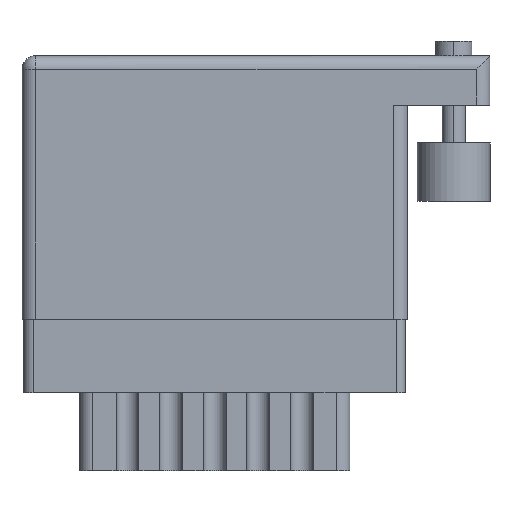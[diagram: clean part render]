
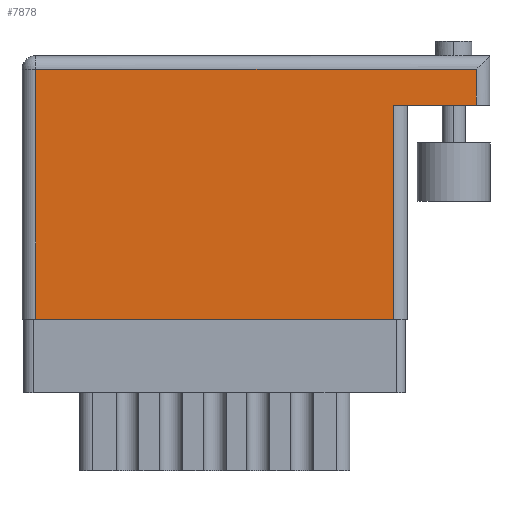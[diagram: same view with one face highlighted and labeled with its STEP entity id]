
A CAD part, front view. The second image highlights one B-rep face of the part: STEP entity #7878.
In plain terms, the highlighted face is planar.
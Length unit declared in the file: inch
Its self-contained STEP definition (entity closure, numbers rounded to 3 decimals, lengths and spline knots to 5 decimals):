
#89 = EDGE_CURVE ( 'NONE', #20875, #8784, #2926, .T. ) ;
#246 = DIRECTION ( 'NONE',  ( 0., 1., 0. ) ) ;
#367 = ORIENTED_EDGE ( 'NONE', *, *, #19739, .T. ) ;
#633 = DIRECTION ( 'NONE',  ( -1., 0., 0. ) ) ;
#801 = VERTEX_POINT ( 'NONE', #1222 ) ;
#1222 = CARTESIAN_POINT ( 'NONE',  ( 1.278, 0.736, 0. ) ) ;
#1273 = ORIENTED_EDGE ( 'NONE', *, *, #17469, .T. ) ;
#1598 = CARTESIAN_POINT ( 'NONE',  ( 0.047, 0., 0. ) ) ;
#1721 = PLANE ( 'NONE',  #6957 ) ;
#2618 = CARTESIAN_POINT ( 'NONE',  ( 1.562, 0.906, 0. ) ) ;
#2769 = ORIENTED_EDGE ( 'NONE', *, *, #17808, .F. ) ;
#2926 = LINE ( 'NONE', #9479, #5356 ) ;
#3146 = CARTESIAN_POINT ( 'NONE',  ( 0., 0.906, 0. ) ) ;
#3317 = LINE ( 'NONE', #13212, #9660 ) ;
#3412 = EDGE_LOOP ( 'NONE', ( #14380, #13756, #2769, #1273, #367, #15903 ) ) ;
#3802 = CARTESIAN_POINT ( 'NONE',  ( 1.278, 0.736, 0. ) ) ;
#4926 = CARTESIAN_POINT ( 'NONE',  ( 1.278, 0., 0. ) ) ;
#5356 = VECTOR ( 'NONE', #16052, 39.37008 ) ;
#6487 = DIRECTION ( 'NONE',  ( 0., 0., -1. ) ) ;
#6518 = VERTEX_POINT ( 'NONE', #19277 ) ;
#6727 = LINE ( 'NONE', #3802, #10354 ) ;
#6957 = AXIS2_PLACEMENT_3D ( 'NONE', #3146, #6487, #16679 ) ;
#7878 = ADVANCED_FACE ( 'NONE', ( #8211 ), #1721, .F. ) ;
#8211 = FACE_OUTER_BOUND ( 'NONE', #3412, .T. ) ;
#8784 = VERTEX_POINT ( 'NONE', #4926 ) ;
#8839 = LINE ( 'NONE', #10759, #20341 ) ;
#9003 = CARTESIAN_POINT ( 'NONE',  ( 1.562, 0.859, 0. ) ) ;
#9479 = CARTESIAN_POINT ( 'NONE',  ( 0., 0., 0. ) ) ;
#9660 = VECTOR ( 'NONE', #14621, 39.37008 ) ;
#10354 = VECTOR ( 'NONE', #246, 39.37008 ) ;
#10759 = CARTESIAN_POINT ( 'NONE',  ( 1.609, 0.736, 0. ) ) ;
#12971 = CARTESIAN_POINT ( 'NONE',  ( 0.047, 0.859, 0. ) ) ;
#13212 = CARTESIAN_POINT ( 'NONE',  ( 0.047, 0., 0. ) ) ;
#13756 = ORIENTED_EDGE ( 'NONE', *, *, #17197, .T. ) ;
#13985 = VECTOR ( 'NONE', #16645, 39.37008 ) ;
#14380 = ORIENTED_EDGE ( 'NONE', *, *, #89, .T. ) ;
#14621 = DIRECTION ( 'NONE',  ( 0., -1., 0. ) ) ;
#15524 = EDGE_CURVE ( 'NONE', #20606, #20875, #3317, .T. ) ;
#15529 = DIRECTION ( 'NONE',  ( 0., 1., 0. ) ) ;
#15903 = ORIENTED_EDGE ( 'NONE', *, *, #15524, .T. ) ;
#16052 = DIRECTION ( 'NONE',  ( 1., 0., 0. ) ) ;
#16544 = CARTESIAN_POINT ( 'NONE',  ( 0., 0.859, 0. ) ) ;
#16645 = DIRECTION ( 'NONE',  ( -1., 0., 0. ) ) ;
#16679 = DIRECTION ( 'NONE',  ( -1., 0., 0. ) ) ;
#17197 = EDGE_CURVE ( 'NONE', #8784, #801, #6727, .T. ) ;
#17469 = EDGE_CURVE ( 'NONE', #6518, #19831, #18869, .T. ) ;
#17808 = EDGE_CURVE ( 'NONE', #6518, #801, #8839, .T. ) ;
#18869 = LINE ( 'NONE', #2618, #19996 ) ;
#19277 = CARTESIAN_POINT ( 'NONE',  ( 1.562, 0.736, 0. ) ) ;
#19739 = EDGE_CURVE ( 'NONE', #19831, #20606, #19982, .T. ) ;
#19831 = VERTEX_POINT ( 'NONE', #9003 ) ;
#19982 = LINE ( 'NONE', #16544, #13985 ) ;
#19996 = VECTOR ( 'NONE', #15529, 39.37008 ) ;
#20341 = VECTOR ( 'NONE', #633, 39.37008 ) ;
#20606 = VERTEX_POINT ( 'NONE', #12971 ) ;
#20875 = VERTEX_POINT ( 'NONE', #1598 ) ;
